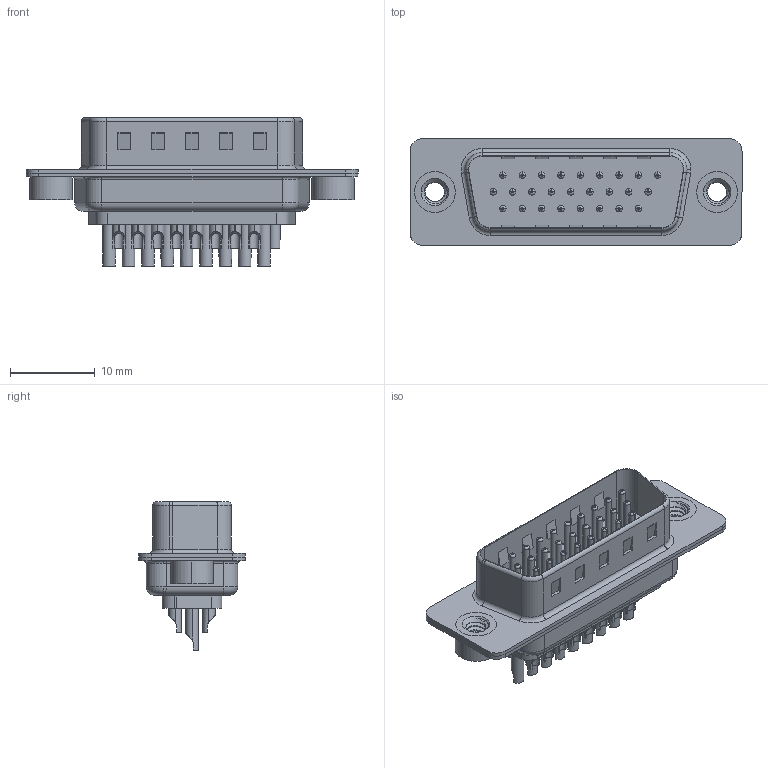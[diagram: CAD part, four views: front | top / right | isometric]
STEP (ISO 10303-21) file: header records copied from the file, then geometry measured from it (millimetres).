
FILE_DESCRIPTION (( 'STEP AP203' ), '1' );
FILE_NAME ('637-026-332-262.STEP', '2020-07-18T01:06:13', ( '' ), ( '' ), 'SwSTEP 2.0', 'SolidWorks 2020', '' );
FILE_SCHEMA (( 'CONFIG_CONTROL_DESIGN' ));
Length unit declared in the file: millimetre
Products named in the file (8): 637-026-332-262; 637 Shell Rear_26 Contacts; 637 Contact Row 2_32; 637 4-40 Threaded Rivet; 637 Contact Row 1_32; 637 Contact Row 3_32; 637 Housing_26 Contacts; 637 Shell Front_26 Contacts
Assembly tree (31 placements, depth 2):
  637-026-332-262
    637 Housing_26 Contacts
    637 Shell Front_26 Contacts
    637 Shell Rear_26 Contacts
    637 Contact Row 1_32  x9
    637 Contact Row 2_32  x9
    637 Contact Row 3_32  x8
    637 4-40 Threaded Rivet  x2
Bounding box: 39.2 x 12.6 x 17.55 mm (x, y, z)
Volume: 1855.6 mm3; surface area: 6927.3 mm2
Topology: 31 solids, 31 shells, 2004 faces, 5121 edges, 3242 vertices
Faces by surface type: cylinder 887, torus 596, plane 503, cone 12, bspline 6
Entity records: 23630 total; most frequent: CARTESIAN_POINT 5138, DIRECTION 3872, ORIENTED_EDGE 3364, EDGE_CURVE 1682, AXIS2_PLACEMENT_3D 1559, VERTEX_POINT 1074, CIRCLE 845, EDGE_LOOP 830
